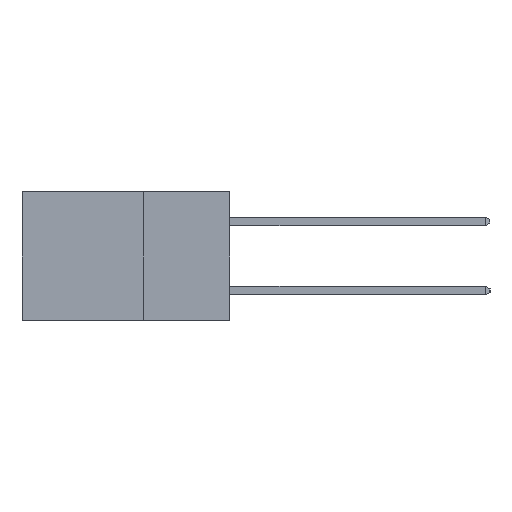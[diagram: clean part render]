
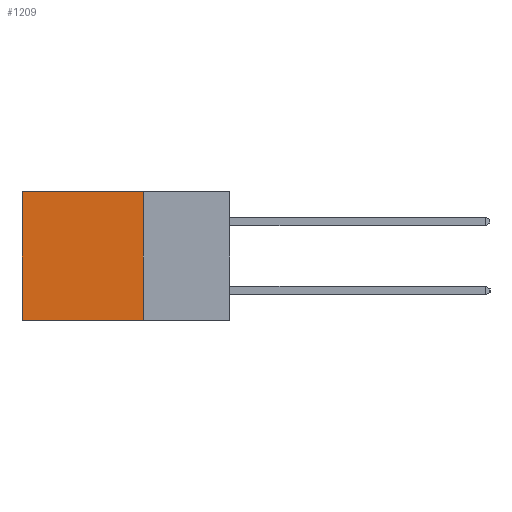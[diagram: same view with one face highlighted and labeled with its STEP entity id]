
A CAD part, left-side view. The second image highlights one B-rep face of the part: STEP entity #1209.
In plain terms, the highlighted planar face has unit normal (-1, 0, 0).
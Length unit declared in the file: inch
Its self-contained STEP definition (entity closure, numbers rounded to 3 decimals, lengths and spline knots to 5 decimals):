
#187 = DIRECTION ( 'NONE',  ( 1., 0., 0. ) ) ;
#1207 = DIRECTION ( 'NONE',  ( 0., 0., -1. ) ) ;
#1209 = ADVANCED_FACE ( 'NONE', ( #1539 ), #1402, .F. ) ;
#1402 = PLANE ( 'NONE',  #24608 ) ;
#1539 = FACE_OUTER_BOUND ( 'NONE', #11010, .T. ) ;
#3026 = CARTESIAN_POINT ( 'NONE',  ( 0.2615, 0.25, -0.37 ) ) ;
#3036 = ORIENTED_EDGE ( 'NONE', *, *, #20807, .F. ) ;
#3906 = CARTESIAN_POINT ( 'NONE',  ( 0.2615, 0.25, 0. ) ) ;
#6065 = CARTESIAN_POINT ( 'NONE',  ( 0.2615, 0.6, -0.37 ) ) ;
#6110 = DIRECTION ( 'NONE',  ( 0., 1., 0. ) ) ;
#6265 = EDGE_CURVE ( 'NONE', #16505, #6862, #9728, .T. ) ;
#6301 = VECTOR ( 'NONE', #16335, 39.37008 ) ;
#6862 = VERTEX_POINT ( 'NONE', #19562 ) ;
#6934 = LINE ( 'NONE', #14343, #6301 ) ;
#8693 = ORIENTED_EDGE ( 'NONE', *, *, #6265, .T. ) ;
#9728 = LINE ( 'NONE', #3906, #25437 ) ;
#10007 = CARTESIAN_POINT ( 'NONE',  ( 0.2615, 0.25, 0. ) ) ;
#10863 = VERTEX_POINT ( 'NONE', #3026 ) ;
#11010 = EDGE_LOOP ( 'NONE', ( #22706, #3036, #15945, #8693 ) ) ;
#12783 = VERTEX_POINT ( 'NONE', #6065 ) ;
#14118 = CARTESIAN_POINT ( 'NONE',  ( 0.2615, 0.25, -0.37 ) ) ;
#14343 = CARTESIAN_POINT ( 'NONE',  ( 0.2615, 0.25, -0.37 ) ) ;
#15294 = CARTESIAN_POINT ( 'NONE',  ( 0.2615, 0.6, -0.37 ) ) ;
#15859 = DIRECTION ( 'NONE',  ( 0., 1., 0. ) ) ;
#15945 = ORIENTED_EDGE ( 'NONE', *, *, #24252, .F. ) ;
#16335 = DIRECTION ( 'NONE',  ( 0., 0., -1. ) ) ;
#16387 = LINE ( 'NONE', #15294, #21642 ) ;
#16505 = VERTEX_POINT ( 'NONE', #10007 ) ;
#19562 = CARTESIAN_POINT ( 'NONE',  ( 0.2615, 0.6, 0. ) ) ;
#19827 = VECTOR ( 'NONE', #6110, 39.37008 ) ;
#20807 = EDGE_CURVE ( 'NONE', #10863, #12783, #25612, .T. ) ;
#21193 = EDGE_CURVE ( 'NONE', #6862, #12783, #16387, .T. ) ;
#21402 = CARTESIAN_POINT ( 'NONE',  ( 0.2615, 0.25, -0.37 ) ) ;
#21642 = VECTOR ( 'NONE', #1207, 39.37008 ) ;
#22097 = DIRECTION ( 'NONE',  ( 0., 0., -1. ) ) ;
#22706 = ORIENTED_EDGE ( 'NONE', *, *, #21193, .T. ) ;
#24252 = EDGE_CURVE ( 'NONE', #16505, #10863, #6934, .T. ) ;
#24608 = AXIS2_PLACEMENT_3D ( 'NONE', #21402, #187, #22097 ) ;
#25437 = VECTOR ( 'NONE', #15859, 39.37008 ) ;
#25612 = LINE ( 'NONE', #14118, #19827 ) ;
